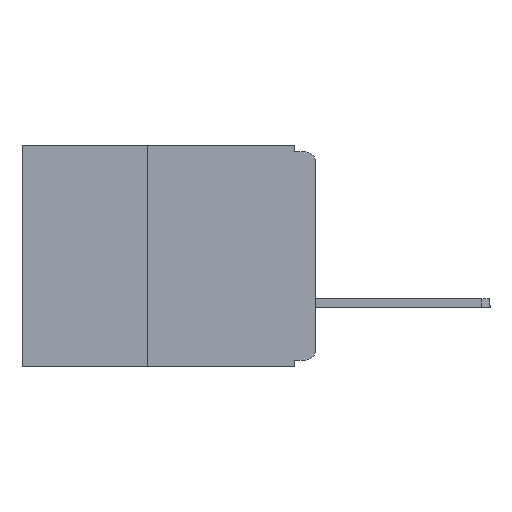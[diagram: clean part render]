
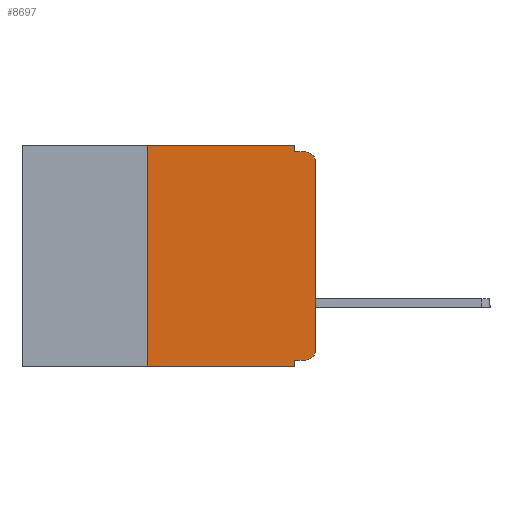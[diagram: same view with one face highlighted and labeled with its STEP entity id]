
A CAD part, left-side view. The second image highlights one B-rep face of the part: STEP entity #8697.
In plain terms, the highlighted planar face has unit normal (-1, 0, 0).
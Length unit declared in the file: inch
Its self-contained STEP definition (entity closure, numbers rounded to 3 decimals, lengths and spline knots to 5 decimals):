
#278 = ORIENTED_EDGE ( 'NONE', *, *, #20336, .F. ) ;
#395 = CARTESIAN_POINT ( 'NONE',  ( 0., 0.437, -0.33 ) ) ;
#876 = AXIS2_PLACEMENT_3D ( 'NONE', #3758, #16049, #7650 ) ;
#918 = ORIENTED_EDGE ( 'NONE', *, *, #19017, .T. ) ;
#1129 = LINE ( 'NONE', #1797, #13426 ) ;
#1326 = VERTEX_POINT ( 'NONE', #17280 ) ;
#1348 = DIRECTION ( 'NONE',  ( 0., -1., 0. ) ) ;
#1445 = VERTEX_POINT ( 'NONE', #6415 ) ;
#1603 = VECTOR ( 'NONE', #1348, 39.37008 ) ;
#1715 = DIRECTION ( 'NONE',  ( 0., 1., 0. ) ) ;
#1732 = CARTESIAN_POINT ( 'NONE',  ( 0., 0.437, 0. ) ) ;
#1797 = CARTESIAN_POINT ( 'NONE',  ( 0., 0.437, 0. ) ) ;
#1995 = ORIENTED_EDGE ( 'NONE', *, *, #2911, .F. ) ;
#2218 = LINE ( 'NONE', #395, #14478 ) ;
#2408 = ORIENTED_EDGE ( 'NONE', *, *, #5320, .F. ) ;
#2488 = ORIENTED_EDGE ( 'NONE', *, *, #11409, .T. ) ;
#2531 = EDGE_CURVE ( 'NONE', #6204, #18224, #4280, .T. ) ;
#2911 = EDGE_CURVE ( 'NONE', #1326, #1445, #16905, .T. ) ;
#3282 = VERTEX_POINT ( 'NONE', #16373 ) ;
#3375 = DIRECTION ( 'NONE',  ( 1., 0., 0. ) ) ;
#3758 = CARTESIAN_POINT ( 'NONE',  ( 0., 0.015, -0.305 ) ) ;
#4032 = ORIENTED_EDGE ( 'NONE', *, *, #12014, .F. ) ;
#4280 = CIRCLE ( 'NONE', #876, 0.015 ) ;
#4534 = ORIENTED_EDGE ( 'NONE', *, *, #20321, .F. ) ;
#4631 = CARTESIAN_POINT ( 'NONE',  ( 0., 0., -0.01 ) ) ;
#5177 = VECTOR ( 'NONE', #20428, 39.37008 ) ;
#5234 = EDGE_LOOP ( 'NONE', ( #2488, #5963, #4032, #1995, #4534, #278, #918, #2408, #6483, #6736 ) ) ;
#5310 = VERTEX_POINT ( 'NONE', #9932 ) ;
#5320 = EDGE_CURVE ( 'NONE', #14150, #17911, #12853, .T. ) ;
#5963 = ORIENTED_EDGE ( 'NONE', *, *, #19531, .T. ) ;
#6204 = VERTEX_POINT ( 'NONE', #6768 ) ;
#6291 = LINE ( 'NONE', #9765, #18418 ) ;
#6415 = CARTESIAN_POINT ( 'NONE',  ( 0., 0.031, -0.01 ) ) ;
#6483 = ORIENTED_EDGE ( 'NONE', *, *, #15088, .F. ) ;
#6570 = CARTESIAN_POINT ( 'NONE',  ( 0., 0., -0.305 ) ) ;
#6732 = DIRECTION ( 'NONE',  ( 0., 0., 1. ) ) ;
#6736 = ORIENTED_EDGE ( 'NONE', *, *, #2531, .T. ) ;
#6761 = VERTEX_POINT ( 'NONE', #17019 ) ;
#6768 = CARTESIAN_POINT ( 'NONE',  ( 0., 0.015, -0.32 ) ) ;
#7650 = DIRECTION ( 'NONE',  ( 0., 0., -1. ) ) ;
#8272 = CIRCLE ( 'NONE', #12053, 0.015 ) ;
#8697 = ADVANCED_FACE ( 'NONE', ( #9999 ), #11392, .F. ) ;
#8896 = CARTESIAN_POINT ( 'NONE',  ( 0., 0.031, -0.32 ) ) ;
#9234 = DIRECTION ( 'NONE',  ( -1., 0., 0. ) ) ;
#9433 = CARTESIAN_POINT ( 'NONE',  ( 0., 0., 0. ) ) ;
#9763 = DIRECTION ( 'NONE',  ( 0., 0., -1. ) ) ;
#9765 = CARTESIAN_POINT ( 'NONE',  ( 0., 0., -0.32 ) ) ;
#9789 = CARTESIAN_POINT ( 'NONE',  ( 0., 0.031, -0.33 ) ) ;
#9932 = CARTESIAN_POINT ( 'NONE',  ( 0., 0.25, 0. ) ) ;
#9999 = FACE_OUTER_BOUND ( 'NONE', #5234, .T. ) ;
#11392 = PLANE ( 'NONE',  #17129 ) ;
#11409 = EDGE_CURVE ( 'NONE', #18224, #13075, #17330, .T. ) ;
#12014 = EDGE_CURVE ( 'NONE', #1445, #3282, #18534, .T. ) ;
#12053 = AXIS2_PLACEMENT_3D ( 'NONE', #18650, #9234, #20233 ) ;
#12772 = VECTOR ( 'NONE', #19044, 39.37008 ) ;
#12853 = LINE ( 'NONE', #9789, #15511 ) ;
#12951 = VECTOR ( 'NONE', #6732, 39.37008 ) ;
#13075 = VERTEX_POINT ( 'NONE', #20354 ) ;
#13382 = CARTESIAN_POINT ( 'NONE',  ( 0., 0.031, 0. ) ) ;
#13426 = VECTOR ( 'NONE', #16120, 39.37008 ) ;
#13599 = CARTESIAN_POINT ( 'NONE',  ( 0., 0.031, -0.33 ) ) ;
#14150 = VERTEX_POINT ( 'NONE', #8896 ) ;
#14478 = VECTOR ( 'NONE', #19478, 39.37008 ) ;
#14525 = DIRECTION ( 'NONE',  ( 0., 0., -1. ) ) ;
#14648 = CARTESIAN_POINT ( 'NONE',  ( 0., 0.25, -0.33 ) ) ;
#15088 = EDGE_CURVE ( 'NONE', #6204, #14150, #6291, .T. ) ;
#15511 = VECTOR ( 'NONE', #9763, 39.37008 ) ;
#16049 = DIRECTION ( 'NONE',  ( -1., 0., 0. ) ) ;
#16120 = DIRECTION ( 'NONE',  ( 0., -1., 0. ) ) ;
#16373 = CARTESIAN_POINT ( 'NONE',  ( 0., 0.015, -0.01 ) ) ;
#16905 = LINE ( 'NONE', #13382, #12772 ) ;
#17019 = CARTESIAN_POINT ( 'NONE',  ( 0., 0.25, -0.33 ) ) ;
#17129 = AXIS2_PLACEMENT_3D ( 'NONE', #1732, #3375, #14525 ) ;
#17280 = CARTESIAN_POINT ( 'NONE',  ( 0., 0.031, 0. ) ) ;
#17330 = LINE ( 'NONE', #9433, #5177 ) ;
#17607 = LINE ( 'NONE', #14648, #12951 ) ;
#17911 = VERTEX_POINT ( 'NONE', #13599 ) ;
#18224 = VERTEX_POINT ( 'NONE', #6570 ) ;
#18418 = VECTOR ( 'NONE', #1715, 39.37008 ) ;
#18534 = LINE ( 'NONE', #4631, #1603 ) ;
#18650 = CARTESIAN_POINT ( 'NONE',  ( 0., 0.015, -0.025 ) ) ;
#19017 = EDGE_CURVE ( 'NONE', #6761, #17911, #2218, .T. ) ;
#19044 = DIRECTION ( 'NONE',  ( 0., 0., -1. ) ) ;
#19478 = DIRECTION ( 'NONE',  ( 0., -1., 0. ) ) ;
#19531 = EDGE_CURVE ( 'NONE', #13075, #3282, #8272, .T. ) ;
#20233 = DIRECTION ( 'NONE',  ( 0., 0., -1. ) ) ;
#20321 = EDGE_CURVE ( 'NONE', #5310, #1326, #1129, .T. ) ;
#20336 = EDGE_CURVE ( 'NONE', #6761, #5310, #17607, .T. ) ;
#20354 = CARTESIAN_POINT ( 'NONE',  ( 0., 0., -0.025 ) ) ;
#20428 = DIRECTION ( 'NONE',  ( 0., 0., 1. ) ) ;
